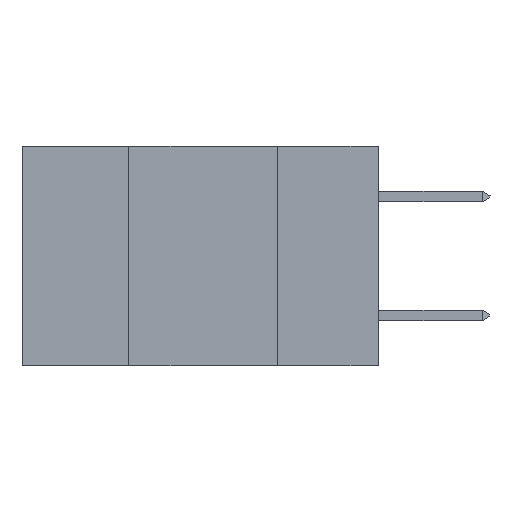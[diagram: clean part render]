
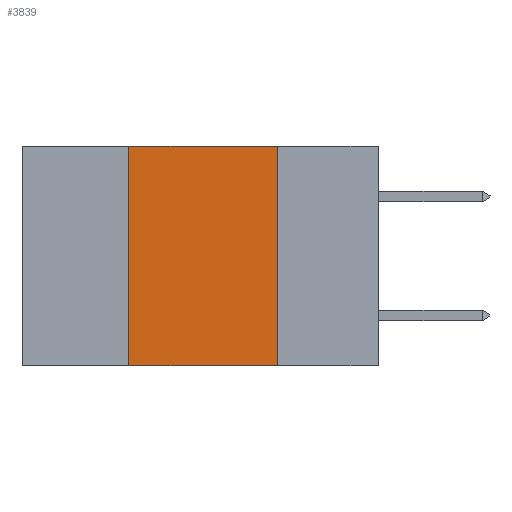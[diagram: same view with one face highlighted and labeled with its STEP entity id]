
A CAD part, left-side view. The second image highlights one B-rep face of the part: STEP entity #3839.
In plain terms, the highlighted planar face has unit normal (-1, 0, 0).
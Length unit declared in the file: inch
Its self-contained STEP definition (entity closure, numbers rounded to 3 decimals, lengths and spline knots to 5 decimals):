
#37 = VECTOR ( 'NONE', #8829, 39.37008 ) ;
#139 = PLANE ( 'NONE',  #11956 ) ;
#495 = ORIENTED_EDGE ( 'NONE', *, *, #16491, .T. ) ;
#949 = VERTEX_POINT ( 'NONE', #1443 ) ;
#1443 = CARTESIAN_POINT ( 'NONE',  ( 0., 0.42, -0.37 ) ) ;
#2534 = EDGE_LOOP ( 'NONE', ( #13972, #13087, #6432, #495 ) ) ;
#3839 = ADVANCED_FACE ( 'NONE', ( #17962 ), #139, .F. ) ;
#4429 = CARTESIAN_POINT ( 'NONE',  ( 0., 0.6, 0. ) ) ;
#5243 = EDGE_CURVE ( 'NONE', #16261, #10481, #7389, .T. ) ;
#5733 = DIRECTION ( 'NONE',  ( 1., 0., 0. ) ) ;
#6393 = CARTESIAN_POINT ( 'NONE',  ( 0., 0.17, -0.37 ) ) ;
#6432 = ORIENTED_EDGE ( 'NONE', *, *, #12610, .F. ) ;
#7088 = LINE ( 'NONE', #8376, #16888 ) ;
#7389 = LINE ( 'NONE', #8855, #9414 ) ;
#8129 = DIRECTION ( 'NONE',  ( 0., 0., -1. ) ) ;
#8376 = CARTESIAN_POINT ( 'NONE',  ( 0., 0.42, -0.37 ) ) ;
#8728 = CARTESIAN_POINT ( 'NONE',  ( 0., 0.6, -0.37 ) ) ;
#8829 = DIRECTION ( 'NONE',  ( 0., -1., 0. ) ) ;
#8855 = CARTESIAN_POINT ( 'NONE',  ( 0., 0.6, 0. ) ) ;
#9121 = VERTEX_POINT ( 'NONE', #9664 ) ;
#9414 = VECTOR ( 'NONE', #12868, 39.37008 ) ;
#9664 = CARTESIAN_POINT ( 'NONE',  ( 0., 0.17, -0.37 ) ) ;
#10399 = LINE ( 'NONE', #8728, #37 ) ;
#10481 = VERTEX_POINT ( 'NONE', #13058 ) ;
#11318 = DIRECTION ( 'NONE',  ( 0., 0., -1. ) ) ;
#11956 = AXIS2_PLACEMENT_3D ( 'NONE', #4429, #5733, #11318 ) ;
#12074 = LINE ( 'NONE', #6393, #12266 ) ;
#12266 = VECTOR ( 'NONE', #8129, 39.37008 ) ;
#12610 = EDGE_CURVE ( 'NONE', #949, #16261, #7088, .T. ) ;
#12868 = DIRECTION ( 'NONE',  ( 0., -1., 0. ) ) ;
#13058 = CARTESIAN_POINT ( 'NONE',  ( 0., 0.17, 0. ) ) ;
#13087 = ORIENTED_EDGE ( 'NONE', *, *, #5243, .F. ) ;
#13870 = EDGE_CURVE ( 'NONE', #10481, #9121, #12074, .T. ) ;
#13972 = ORIENTED_EDGE ( 'NONE', *, *, #13870, .F. ) ;
#15322 = CARTESIAN_POINT ( 'NONE',  ( 0., 0.42, 0. ) ) ;
#15401 = DIRECTION ( 'NONE',  ( 0., 0., 1. ) ) ;
#16261 = VERTEX_POINT ( 'NONE', #15322 ) ;
#16491 = EDGE_CURVE ( 'NONE', #949, #9121, #10399, .T. ) ;
#16888 = VECTOR ( 'NONE', #15401, 39.37008 ) ;
#17962 = FACE_OUTER_BOUND ( 'NONE', #2534, .T. ) ;
